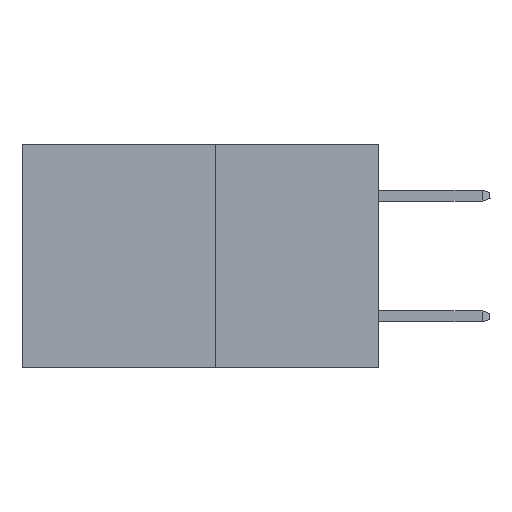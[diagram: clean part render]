
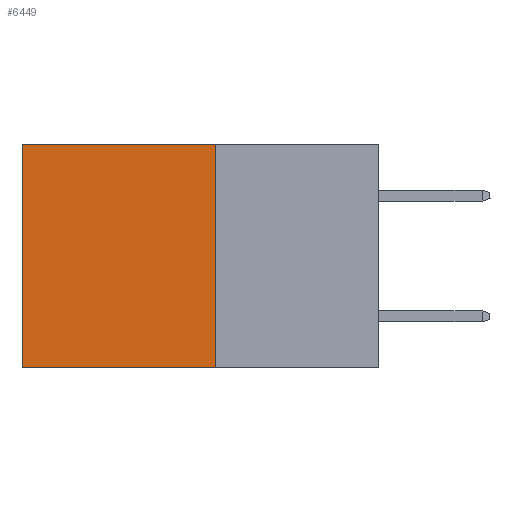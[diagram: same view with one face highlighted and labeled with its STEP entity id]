
A CAD part, left-side view. The second image highlights one B-rep face of the part: STEP entity #6449.
In plain terms, the highlighted planar face has unit normal (-1, 0, 0).
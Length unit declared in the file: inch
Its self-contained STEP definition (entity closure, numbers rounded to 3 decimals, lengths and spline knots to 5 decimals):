
#213 = ORIENTED_EDGE ( 'NONE', *, *, #13788, .T. ) ;
#1629 = VERTEX_POINT ( 'NONE', #2788 ) ;
#2121 = CARTESIAN_POINT ( 'NONE',  ( 0.277, 0.27, -0.37 ) ) ;
#2170 = VECTOR ( 'NONE', #13306, 39.37008 ) ;
#2235 = DIRECTION ( 'NONE',  ( 0., 0., -1. ) ) ;
#2260 = CARTESIAN_POINT ( 'NONE',  ( 0.277, 0.27, -0.37 ) ) ;
#2788 = CARTESIAN_POINT ( 'NONE',  ( 0.277, 0.27, 0. ) ) ;
#3104 = EDGE_CURVE ( 'NONE', #1629, #13193, #3292, .T. ) ;
#3292 = LINE ( 'NONE', #2121, #9748 ) ;
#4300 = FACE_OUTER_BOUND ( 'NONE', #8333, .T. ) ;
#4483 = DIRECTION ( 'NONE',  ( 0., 0., -1. ) ) ;
#4558 = EDGE_CURVE ( 'NONE', #16218, #13078, #9710, .T. ) ;
#4661 = DIRECTION ( 'NONE',  ( 1., 0., 0. ) ) ;
#5637 = EDGE_CURVE ( 'NONE', #13193, #13078, #5842, .T. ) ;
#5842 = LINE ( 'NONE', #2260, #2170 ) ;
#6449 = ADVANCED_FACE ( 'NONE', ( #4300 ), #15752, .F. ) ;
#7242 = DIRECTION ( 'NONE',  ( 0., 1., 0. ) ) ;
#8199 = VECTOR ( 'NONE', #7242, 39.37008 ) ;
#8333 = EDGE_LOOP ( 'NONE', ( #15170, #12764, #14622, #213 ) ) ;
#9662 = CARTESIAN_POINT ( 'NONE',  ( 0.277, 0.27, -0.37 ) ) ;
#9710 = LINE ( 'NONE', #11856, #16582 ) ;
#9748 = VECTOR ( 'NONE', #2235, 39.37008 ) ;
#11382 = CARTESIAN_POINT ( 'NONE',  ( 0.277, 0.59, 0. ) ) ;
#11463 = DIRECTION ( 'NONE',  ( 0., 0., -1. ) ) ;
#11856 = CARTESIAN_POINT ( 'NONE',  ( 0.277, 0.59, -0.37 ) ) ;
#12764 = ORIENTED_EDGE ( 'NONE', *, *, #5637, .F. ) ;
#13078 = VERTEX_POINT ( 'NONE', #15958 ) ;
#13193 = VERTEX_POINT ( 'NONE', #9662 ) ;
#13306 = DIRECTION ( 'NONE',  ( 0., 1., 0. ) ) ;
#13497 = CARTESIAN_POINT ( 'NONE',  ( 0.277, 0.27, 0. ) ) ;
#13683 = AXIS2_PLACEMENT_3D ( 'NONE', #14845, #4661, #11463 ) ;
#13788 = EDGE_CURVE ( 'NONE', #1629, #16218, #15951, .T. ) ;
#14622 = ORIENTED_EDGE ( 'NONE', *, *, #3104, .F. ) ;
#14845 = CARTESIAN_POINT ( 'NONE',  ( 0.277, 0.27, -0.37 ) ) ;
#15170 = ORIENTED_EDGE ( 'NONE', *, *, #4558, .T. ) ;
#15752 = PLANE ( 'NONE',  #13683 ) ;
#15951 = LINE ( 'NONE', #13497, #8199 ) ;
#15958 = CARTESIAN_POINT ( 'NONE',  ( 0.277, 0.59, -0.37 ) ) ;
#16218 = VERTEX_POINT ( 'NONE', #11382 ) ;
#16582 = VECTOR ( 'NONE', #4483, 39.37008 ) ;
